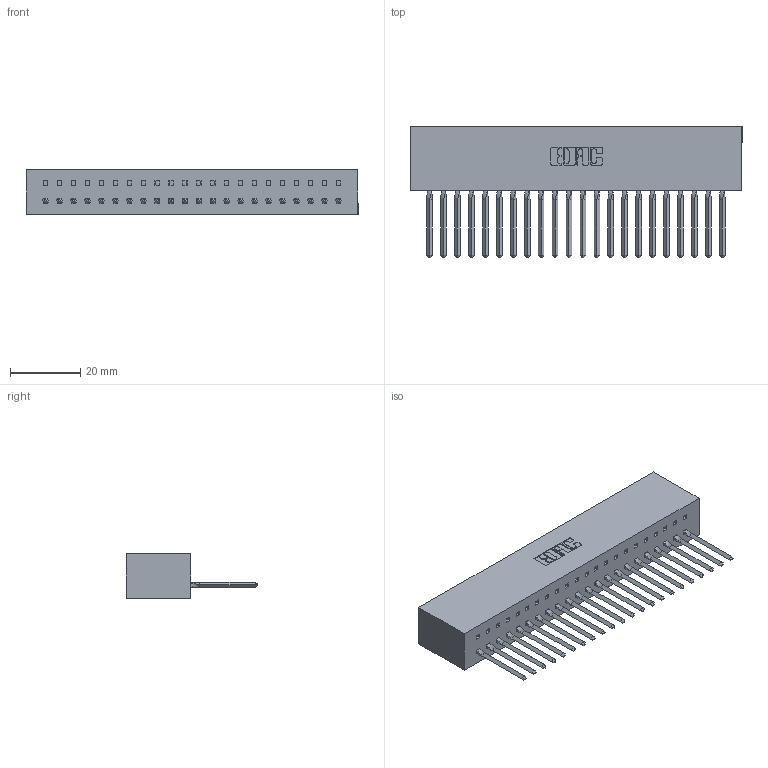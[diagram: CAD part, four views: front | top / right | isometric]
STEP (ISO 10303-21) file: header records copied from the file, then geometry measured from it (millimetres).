
FILE_DESCRIPTION (( 'STEP AP203' ), '1' );
FILE_NAME ('317-022-541-601.STEP', '2020-02-27T17:14:23', ( '' ), ( '' ), 'SwSTEP 2.0', 'SolidWorks 2016', '' );
FILE_SCHEMA (( 'CONFIG_CONTROL_DESIGN' ));
Length unit declared in the file: inch
Products named in the file (3): 317 Part_Lugless; 317-022-541-601; 317-290-002_541
Assembly tree (23 placements, depth 2):
  317-022-541-601
    317 Part_Lugless
    317-290-002_541  x22
Bounding box: 94.39 x 37.34 x 12.7 mm (x, y, z)
Volume: 16397.1 mm3; surface area: 22697.2 mm2
Topology: 23 solids, 23 shells, 3434 faces, 9787 edges, 6362 vertices
Faces by surface type: plane 2778, cylinder 568, bspline 88
Entity records: 35026 total; most frequent: CARTESIAN_POINT 6859, ORIENTED_EDGE 6134, DIRECTION 5015, EDGE_CURVE 3067, LINE 2711, VECTOR 2711, VERTEX_POINT 2036, AXIS2_PLACEMENT_3D 1152
